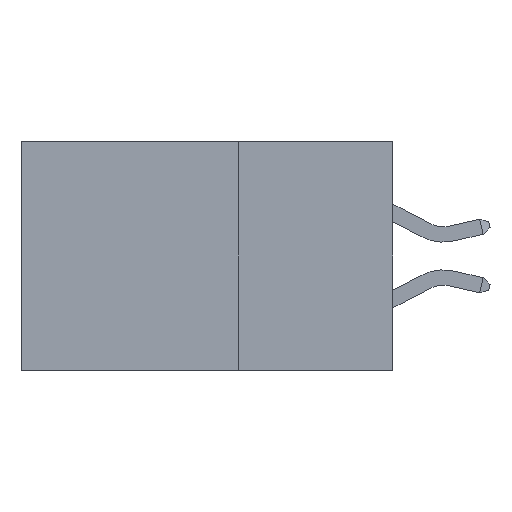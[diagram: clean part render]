
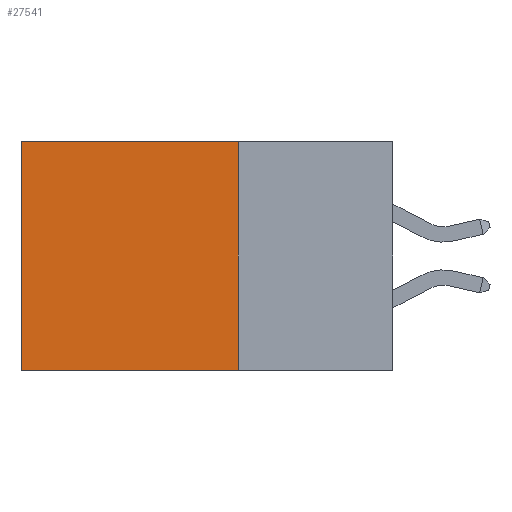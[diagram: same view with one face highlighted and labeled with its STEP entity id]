
A CAD part, left-side view. The second image highlights one B-rep face of the part: STEP entity #27541.
In plain terms, the highlighted planar face has unit normal (-1, 0, 0).
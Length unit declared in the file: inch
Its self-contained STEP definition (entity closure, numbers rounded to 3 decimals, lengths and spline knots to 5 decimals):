
#1542 = PLANE ( 'NONE',  #12235 ) ;
#2357 = VERTEX_POINT ( 'NONE', #25374 ) ;
#3447 = LINE ( 'NONE', #15420, #34145 ) ;
#4360 = DIRECTION ( 'NONE',  ( 1., 0., 0. ) ) ;
#4883 = ORIENTED_EDGE ( 'NONE', *, *, #26402, .F. ) ;
#5393 = CARTESIAN_POINT ( 'NONE',  ( 0.2875, 0.25, 0. ) ) ;
#7180 = CARTESIAN_POINT ( 'NONE',  ( 0.2875, 0.6, 0. ) ) ;
#7773 = ORIENTED_EDGE ( 'NONE', *, *, #33781, .F. ) ;
#8634 = CARTESIAN_POINT ( 'NONE',  ( 0.2875, 0.25, 0. ) ) ;
#11202 = ORIENTED_EDGE ( 'NONE', *, *, #25196, .T. ) ;
#12235 = AXIS2_PLACEMENT_3D ( 'NONE', #20889, #4360, #18222 ) ;
#14674 = VECTOR ( 'NONE', #25421, 39.37008 ) ;
#15420 = CARTESIAN_POINT ( 'NONE',  ( 0.2875, 0.25, 0. ) ) ;
#16808 = LINE ( 'NONE', #8634, #14674 ) ;
#18222 = DIRECTION ( 'NONE',  ( 0., 0., -1. ) ) ;
#20889 = CARTESIAN_POINT ( 'NONE',  ( 0.2875, 0.25, 0. ) ) ;
#21975 = VERTEX_POINT ( 'NONE', #25299 ) ;
#23430 = ORIENTED_EDGE ( 'NONE', *, *, #24529, .T. ) ;
#24529 = EDGE_CURVE ( 'NONE', #34949, #2357, #3447, .T. ) ;
#25196 = EDGE_CURVE ( 'NONE', #2357, #26179, #32856, .T. ) ;
#25299 = CARTESIAN_POINT ( 'NONE',  ( 0.2875, 0.25, -0.37 ) ) ;
#25374 = CARTESIAN_POINT ( 'NONE',  ( 0.2875, 0.6, 0. ) ) ;
#25421 = DIRECTION ( 'NONE',  ( 0., 0., -1. ) ) ;
#26114 = DIRECTION ( 'NONE',  ( 0., 0., -1. ) ) ;
#26179 = VERTEX_POINT ( 'NONE', #34889 ) ;
#26402 = EDGE_CURVE ( 'NONE', #21975, #26179, #30225, .T. ) ;
#27541 = ADVANCED_FACE ( 'NONE', ( #33238 ), #1542, .F. ) ;
#30050 = CARTESIAN_POINT ( 'NONE',  ( 0.2875, 0.25, -0.37 ) ) ;
#30225 = LINE ( 'NONE', #30050, #34972 ) ;
#30690 = VECTOR ( 'NONE', #26114, 39.37008 ) ;
#30953 = EDGE_LOOP ( 'NONE', ( #11202, #4883, #7773, #23430 ) ) ;
#32842 = DIRECTION ( 'NONE',  ( 0., 1., 0. ) ) ;
#32856 = LINE ( 'NONE', #7180, #30690 ) ;
#33238 = FACE_OUTER_BOUND ( 'NONE', #30953, .T. ) ;
#33781 = EDGE_CURVE ( 'NONE', #34949, #21975, #16808, .T. ) ;
#34145 = VECTOR ( 'NONE', #34497, 39.37008 ) ;
#34497 = DIRECTION ( 'NONE',  ( 0., 1., 0. ) ) ;
#34889 = CARTESIAN_POINT ( 'NONE',  ( 0.2875, 0.6, -0.37 ) ) ;
#34949 = VERTEX_POINT ( 'NONE', #5393 ) ;
#34972 = VECTOR ( 'NONE', #32842, 39.37008 ) ;
